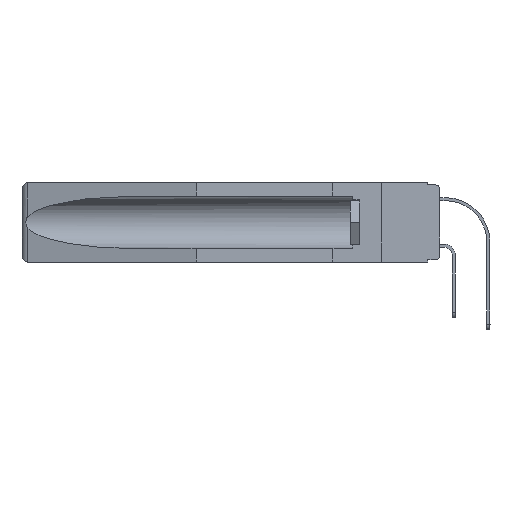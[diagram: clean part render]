
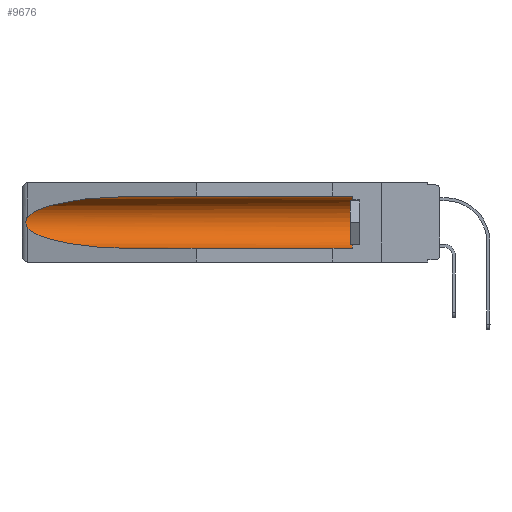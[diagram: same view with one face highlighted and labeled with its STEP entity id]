
A CAD part, left-side view. The second image highlights one B-rep face of the part: STEP entity #9676.
In plain terms, the highlighted cylindrical face has radius 2.857 mm (diameter 5.715 mm), a partial arc.
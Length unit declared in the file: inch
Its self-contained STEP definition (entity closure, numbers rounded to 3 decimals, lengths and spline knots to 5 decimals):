
#704 = CARTESIAN_POINT ( 'NONE',  ( 0.155, 1.07973, -0.059 ) ) ;
#810 = CARTESIAN_POINT ( 'NONE',  ( 0.21114, 1.30732, -0.059 ) ) ;
#1667 = CARTESIAN_POINT ( 'NONE',  ( 0.2673, 1.53269, -0.17917 ) ) ;
#1757 = VECTOR ( 'NONE', #14087, 39.37008 ) ;
#2144 =( BOUNDED_CURVE ( )  B_SPLINE_CURVE ( 3, ( #704, #810, #19574, #11984 ),
 .UNSPECIFIED., .F., .F. ) 
 B_SPLINE_CURVE_WITH_KNOTS ( ( 4, 4 ),
 ( 4.71239, 6.08839 ),
 .UNSPECIFIED. ) 
 CURVE ( )  GEOMETRIC_REPRESENTATION_ITEM ( )  RATIONAL_B_SPLINE_CURVE ( ( 1., 0.848, 0.848, 1. ) ) 
 REPRESENTATION_ITEM ( '' )  );
#2573 = VERTEX_POINT ( 'NONE', #16012 ) ;
#2768 = ORIENTED_EDGE ( 'NONE', *, *, #13769, .T. ) ;
#3240 = CARTESIAN_POINT ( 'NONE',  ( 0.26537, 1.52718, -0.14972 ) ) ;
#3338 = CARTESIAN_POINT ( 'NONE',  ( 0.2673, 1.5327, -0.16383 ) ) ;
#3340 = CARTESIAN_POINT ( 'NONE',  ( 0.155, 0.126, -0.284 ) ) ;
#3565 = CIRCLE ( 'NONE', #13889, 0.1125 ) ;
#4229 = DIRECTION ( 'NONE',  ( 0., 1., 0. ) ) ;
#4276 =( BOUNDED_CURVE ( )  B_SPLINE_CURVE ( 3, ( #6139, #6026, #7385, #20186 ),
 .UNSPECIFIED., .F., .F. ) 
 B_SPLINE_CURVE_WITH_KNOTS ( ( 4, 4 ),
 ( 0.1948, 1.5708 ),
 .UNSPECIFIED. ) 
 CURVE ( )  GEOMETRIC_REPRESENTATION_ITEM ( )  RATIONAL_B_SPLINE_CURVE ( ( 1., 0.848, 0.848, 1. ) ) 
 REPRESENTATION_ITEM ( '' )  );
#4357 = VERTEX_POINT ( 'NONE', #20561 ) ;
#4454 = CARTESIAN_POINT ( 'NONE',  ( 0.155, -0.30754, -0.1715 ) ) ;
#4835 = CARTESIAN_POINT ( 'NONE',  ( 0.155, 0.126, -0.059 ) ) ;
#5164 = ORIENTED_EDGE ( 'NONE', *, *, #17952, .F. ) ;
#5916 = DIRECTION ( 'NONE',  ( 0., 0., 1. ) ) ;
#6026 = CARTESIAN_POINT ( 'NONE',  ( 0.25451, 1.48313, -0.24835 ) ) ;
#6056 = ORIENTED_EDGE ( 'NONE', *, *, #12847, .T. ) ;
#6139 = CARTESIAN_POINT ( 'NONE',  ( 0.26537, 1.52718, -0.19328 ) ) ;
#7385 = CARTESIAN_POINT ( 'NONE',  ( 0.21114, 1.30732, -0.284 ) ) ;
#7622 = CARTESIAN_POINT ( 'NONE',  ( 0.155, -0.30754, -0.284 ) ) ;
#7946 = CARTESIAN_POINT ( 'NONE',  ( 0.26597, 1.5296, -0.19026 ) ) ;
#8039 = CARTESIAN_POINT ( 'NONE',  ( 0.26537, 1.52718, -0.19328 ) ) ;
#8335 = CARTESIAN_POINT ( 'NONE',  ( 0.26537, 1.52718, -0.19328 ) ) ;
#8389 = VERTEX_POINT ( 'NONE', #8335 ) ;
#9498 = CARTESIAN_POINT ( 'NONE',  ( 0.26655, 1.53094, -0.18657 ) ) ;
#9587 = AXIS2_PLACEMENT_3D ( 'NONE', #4454, #15614, #5916 ) ;
#9606 = CARTESIAN_POINT ( 'NONE',  ( 0.2675, 1.53308, -0.16763 ) ) ;
#9676 = ADVANCED_FACE ( 'NONE', ( #20175 ), #10501, .F. ) ;
#10230 = DIRECTION ( 'NONE',  ( 0., 0., 1. ) ) ;
#10298 = B_SPLINE_CURVE_WITH_KNOTS ( 'NONE', 3,
 ( #3240, #17521, #19174, #3338, #9606, #18869, #1667, #9498, #7946, #8039 ),
 .UNSPECIFIED., .F., .F.,
 ( 4, 2, 2, 2, 4 ),
 ( 0., 0.00029, 0.00058, 0.00087, 0.00117 ),
 .UNSPECIFIED. ) ;
#10501 = CYLINDRICAL_SURFACE ( 'NONE', #9587, 0.1125 ) ;
#10502 = EDGE_CURVE ( 'NONE', #14923, #15779, #3565, .T. ) ;
#10881 = EDGE_CURVE ( 'NONE', #2573, #17270, #2144, .T. ) ;
#11100 = EDGE_CURVE ( 'NONE', #8389, #4357, #4276, .T. ) ;
#11243 = ORIENTED_EDGE ( 'NONE', *, *, #10881, .T. ) ;
#11741 = ORIENTED_EDGE ( 'NONE', *, *, #10502, .T. ) ;
#11984 = CARTESIAN_POINT ( 'NONE',  ( 0.26537, 1.52718, -0.14972 ) ) ;
#12162 = LINE ( 'NONE', #14047, #13257 ) ;
#12835 = EDGE_LOOP ( 'NONE', ( #11243, #2768, #17364, #5164, #11741, #6056 ) ) ;
#12847 = EDGE_CURVE ( 'NONE', #15779, #2573, #12162, .T. ) ;
#13257 = VECTOR ( 'NONE', #4229, 39.37008 ) ;
#13769 = EDGE_CURVE ( 'NONE', #17270, #8389, #10298, .T. ) ;
#13889 = AXIS2_PLACEMENT_3D ( 'NONE', #18148, #20001, #10230 ) ;
#14047 = CARTESIAN_POINT ( 'NONE',  ( 0.155, -0.30754, -0.059 ) ) ;
#14087 = DIRECTION ( 'NONE',  ( 0., 1., 0. ) ) ;
#14923 = VERTEX_POINT ( 'NONE', #3340 ) ;
#15612 = CARTESIAN_POINT ( 'NONE',  ( 0.26537, 1.52718, -0.14972 ) ) ;
#15614 = DIRECTION ( 'NONE',  ( 0., 1., 0. ) ) ;
#15779 = VERTEX_POINT ( 'NONE', #4835 ) ;
#16012 = CARTESIAN_POINT ( 'NONE',  ( 0.155, 1.07973, -0.059 ) ) ;
#17094 = LINE ( 'NONE', #7622, #1757 ) ;
#17270 = VERTEX_POINT ( 'NONE', #15612 ) ;
#17364 = ORIENTED_EDGE ( 'NONE', *, *, #11100, .T. ) ;
#17521 = CARTESIAN_POINT ( 'NONE',  ( 0.26597, 1.52961, -0.15275 ) ) ;
#17952 = EDGE_CURVE ( 'NONE', #14923, #4357, #17094, .T. ) ;
#18148 = CARTESIAN_POINT ( 'NONE',  ( 0.155, 0.126, -0.1715 ) ) ;
#18869 = CARTESIAN_POINT ( 'NONE',  ( 0.2675, 1.53308, -0.17534 ) ) ;
#19174 = CARTESIAN_POINT ( 'NONE',  ( 0.26654, 1.53092, -0.15636 ) ) ;
#19574 = CARTESIAN_POINT ( 'NONE',  ( 0.25451, 1.48313, -0.09465 ) ) ;
#20001 = DIRECTION ( 'NONE',  ( 0., -1., 0. ) ) ;
#20175 = FACE_OUTER_BOUND ( 'NONE', #12835, .T. ) ;
#20186 = CARTESIAN_POINT ( 'NONE',  ( 0.155, 1.07973, -0.284 ) ) ;
#20561 = CARTESIAN_POINT ( 'NONE',  ( 0.155, 1.07973, -0.284 ) ) ;
